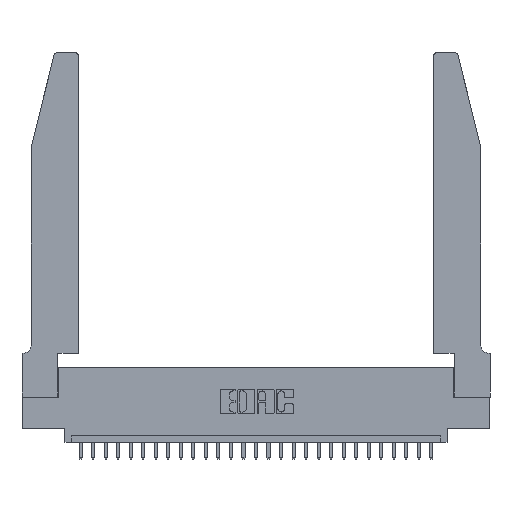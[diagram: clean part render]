
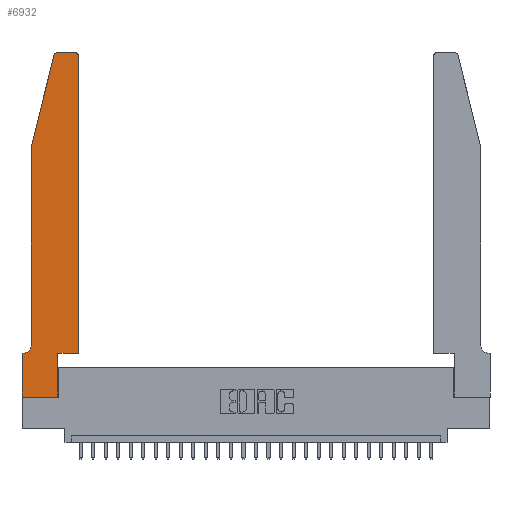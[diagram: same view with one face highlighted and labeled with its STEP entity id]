
A CAD part, top view. The second image highlights one B-rep face of the part: STEP entity #6932.
In plain terms, the highlighted planar face has unit normal (0, 0, 1).
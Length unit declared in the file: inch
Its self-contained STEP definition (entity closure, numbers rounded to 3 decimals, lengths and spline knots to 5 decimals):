
#98 = LINE ( 'NONE', #25746, #4545 ) ;
#284 = CIRCLE ( 'NONE', #2740, 0.07 ) ;
#469 = VERTEX_POINT ( 'NONE', #4479 ) ;
#499 = CIRCLE ( 'NONE', #12486, 0.03 ) ;
#538 = DIRECTION ( 'NONE',  ( 0., 1., 0. ) ) ;
#573 = VECTOR ( 'NONE', #15746, 39.37008 ) ;
#632 = VERTEX_POINT ( 'NONE', #27922 ) ;
#677 = CARTESIAN_POINT ( 'NONE',  ( 0.2865, 0., 0.37 ) ) ;
#1033 = VECTOR ( 'NONE', #1389, 39.37008 ) ;
#1291 = CARTESIAN_POINT ( 'NONE',  ( 0., 0., 0.37 ) ) ;
#1308 = ORIENTED_EDGE ( 'NONE', *, *, #15383, .T. ) ;
#1389 = DIRECTION ( 'NONE',  ( 0., -1., 0. ) ) ;
#1395 = LINE ( 'NONE', #14197, #15892 ) ;
#2292 = ORIENTED_EDGE ( 'NONE', *, *, #10619, .T. ) ;
#2417 = CARTESIAN_POINT ( 'NONE',  ( 0.284, 2.72, 0.37 ) ) ;
#2649 = DIRECTION ( 'NONE',  ( 0., -1., 0. ) ) ;
#2657 = LINE ( 'NONE', #26398, #573 ) ;
#2740 = AXIS2_PLACEMENT_3D ( 'NONE', #25289, #16289, #8616 ) ;
#3083 = AXIS2_PLACEMENT_3D ( 'NONE', #3349, #16385, #27313 ) ;
#3349 = CARTESIAN_POINT ( 'NONE',  ( 0., 0.35, 0.37 ) ) ;
#4479 = CARTESIAN_POINT ( 'NONE',  ( 0.25487, 2.72718, 0.37 ) ) ;
#4545 = VECTOR ( 'NONE', #27950, 39.37008 ) ;
#4748 = ORIENTED_EDGE ( 'NONE', *, *, #19093, .T. ) ;
#5594 = VERTEX_POINT ( 'NONE', #677 ) ;
#5824 = FACE_OUTER_BOUND ( 'NONE', #18895, .T. ) ;
#5904 = CARTESIAN_POINT ( 'NONE',  ( 0.0755, 0.42, 0.37 ) ) ;
#6151 = CARTESIAN_POINT ( 'NONE',  ( 0.2865, 0.35, 0.37 ) ) ;
#6912 = CARTESIAN_POINT ( 'NONE',  ( 0.0755, 0.35, 0.37 ) ) ;
#6932 = ADVANCED_FACE ( 'NONE', ( #5824 ), #23093, .T. ) ;
#7604 = EDGE_CURVE ( 'NONE', #469, #17773, #22315, .T. ) ;
#7853 = VERTEX_POINT ( 'NONE', #11760 ) ;
#8605 = DIRECTION ( 'NONE',  ( 1., 0., 0. ) ) ;
#8616 = DIRECTION ( 'NONE',  ( -1., 0., 0. ) ) ;
#8755 = LINE ( 'NONE', #6912, #15321 ) ;
#8939 = VECTOR ( 'NONE', #16364, 39.37008 ) ;
#9167 = ORIENTED_EDGE ( 'NONE', *, *, #10585, .T. ) ;
#9282 = DIRECTION ( 'NONE',  ( -1., 0., 0. ) ) ;
#9583 = CARTESIAN_POINT ( 'NONE',  ( 0.284, 2.75, 0.37 ) ) ;
#9973 = CIRCLE ( 'NONE', #12933, 0.03 ) ;
#10018 = VERTEX_POINT ( 'NONE', #25868 ) ;
#10585 = EDGE_CURVE ( 'NONE', #10018, #11257, #13432, .T. ) ;
#10619 = EDGE_CURVE ( 'NONE', #11257, #469, #9973, .T. ) ;
#11257 = VERTEX_POINT ( 'NONE', #9583 ) ;
#11760 = CARTESIAN_POINT ( 'NONE',  ( 0., 0.35, 0.37 ) ) ;
#12337 = VERTEX_POINT ( 'NONE', #13490 ) ;
#12486 = AXIS2_PLACEMENT_3D ( 'NONE', #19138, #25751, #19239 ) ;
#12586 = VECTOR ( 'NONE', #20043, 39.37008 ) ;
#12933 = AXIS2_PLACEMENT_3D ( 'NONE', #2417, #28495, #8605 ) ;
#13105 = LINE ( 'NONE', #1291, #1033 ) ;
#13432 = LINE ( 'NONE', #20493, #8939 ) ;
#13490 = CARTESIAN_POINT ( 'NONE',  ( 0.0055, 0.35, 0.37 ) ) ;
#13651 = CARTESIAN_POINT ( 'NONE',  ( 0.0755, 2., 0.37 ) ) ;
#14183 = EDGE_CURVE ( 'NONE', #12337, #7853, #8755, .T. ) ;
#14197 = CARTESIAN_POINT ( 'NONE',  ( 0.2865, 0.35, 0.37 ) ) ;
#14697 = VECTOR ( 'NONE', #2649, 39.37008 ) ;
#15119 = ORIENTED_EDGE ( 'NONE', *, *, #27150, .T. ) ;
#15321 = VECTOR ( 'NONE', #9282, 39.37008 ) ;
#15383 = EDGE_CURVE ( 'NONE', #632, #5594, #98, .T. ) ;
#15455 = VECTOR ( 'NONE', #23470, 39.37008 ) ;
#15746 = DIRECTION ( 'NONE',  ( 1., 0., 0. ) ) ;
#15892 = VECTOR ( 'NONE', #538, 39.37008 ) ;
#16018 = LINE ( 'NONE', #17296, #12586 ) ;
#16289 = DIRECTION ( 'NONE',  ( 0., 0., -1. ) ) ;
#16364 = DIRECTION ( 'NONE',  ( -1., 0., 0. ) ) ;
#16385 = DIRECTION ( 'NONE',  ( 0., 0., 1. ) ) ;
#16455 = ORIENTED_EDGE ( 'NONE', *, *, #17836, .T. ) ;
#16694 = ORIENTED_EDGE ( 'NONE', *, *, #28045, .T. ) ;
#16830 = CARTESIAN_POINT ( 'NONE',  ( 0.0755, 2., 0.37 ) ) ;
#17263 = EDGE_CURVE ( 'NONE', #5594, #18409, #1395, .T. ) ;
#17296 = CARTESIAN_POINT ( 'NONE',  ( 0.4505, 0.35, 0.37 ) ) ;
#17343 = VERTEX_POINT ( 'NONE', #22087 ) ;
#17773 = VERTEX_POINT ( 'NONE', #21440 ) ;
#17836 = EDGE_CURVE ( 'NONE', #7853, #632, #13105, .T. ) ;
#18409 = VERTEX_POINT ( 'NONE', #6151 ) ;
#18677 = ORIENTED_EDGE ( 'NONE', *, *, #17263, .T. ) ;
#18895 = EDGE_LOOP ( 'NONE', ( #9167, #2292, #25214, #15119, #19038, #27115, #16455, #1308, #18677, #4748, #16694, #21278 ) ) ;
#19038 = ORIENTED_EDGE ( 'NONE', *, *, #25951, .T. ) ;
#19093 = EDGE_CURVE ( 'NONE', #18409, #17343, #2657, .T. ) ;
#19138 = CARTESIAN_POINT ( 'NONE',  ( 0.4205, 2.72, 0.37 ) ) ;
#19239 = DIRECTION ( 'NONE',  ( 1., 0., 0. ) ) ;
#19972 = CARTESIAN_POINT ( 'NONE',  ( 0.4505, 2.72, 0.37 ) ) ;
#20043 = DIRECTION ( 'NONE',  ( 0., 1., 0. ) ) ;
#20044 = EDGE_CURVE ( 'NONE', #27636, #10018, #499, .T. ) ;
#20493 = CARTESIAN_POINT ( 'NONE',  ( 0.2605, 2.75, 0.37 ) ) ;
#21278 = ORIENTED_EDGE ( 'NONE', *, *, #20044, .T. ) ;
#21440 = CARTESIAN_POINT ( 'NONE',  ( 0.0755, 2., 0.37 ) ) ;
#22087 = CARTESIAN_POINT ( 'NONE',  ( 0.4505, 0.35, 0.37 ) ) ;
#22315 = LINE ( 'NONE', #16830, #15455 ) ;
#23093 = PLANE ( 'NONE',  #3083 ) ;
#23294 = LINE ( 'NONE', #13651, #14697 ) ;
#23470 = DIRECTION ( 'NONE',  ( -0.239, -0.971, 0. ) ) ;
#25214 = ORIENTED_EDGE ( 'NONE', *, *, #7604, .T. ) ;
#25289 = CARTESIAN_POINT ( 'NONE',  ( 0.0055, 0.42, 0.37 ) ) ;
#25746 = CARTESIAN_POINT ( 'NONE',  ( 0., 0., 0.37 ) ) ;
#25751 = DIRECTION ( 'NONE',  ( 0., 0., 1. ) ) ;
#25868 = CARTESIAN_POINT ( 'NONE',  ( 0.4205, 2.75, 0.37 ) ) ;
#25951 = EDGE_CURVE ( 'NONE', #27956, #12337, #284, .T. ) ;
#26398 = CARTESIAN_POINT ( 'NONE',  ( 0.4505, 0.35, 0.37 ) ) ;
#27115 = ORIENTED_EDGE ( 'NONE', *, *, #14183, .T. ) ;
#27150 = EDGE_CURVE ( 'NONE', #17773, #27956, #23294, .T. ) ;
#27313 = DIRECTION ( 'NONE',  ( 1., 0., 0. ) ) ;
#27636 = VERTEX_POINT ( 'NONE', #19972 ) ;
#27922 = CARTESIAN_POINT ( 'NONE',  ( 0., 0., 0.37 ) ) ;
#27950 = DIRECTION ( 'NONE',  ( 1., 0., 0. ) ) ;
#27956 = VERTEX_POINT ( 'NONE', #5904 ) ;
#28045 = EDGE_CURVE ( 'NONE', #17343, #27636, #16018, .T. ) ;
#28495 = DIRECTION ( 'NONE',  ( 0., 0., 1. ) ) ;
